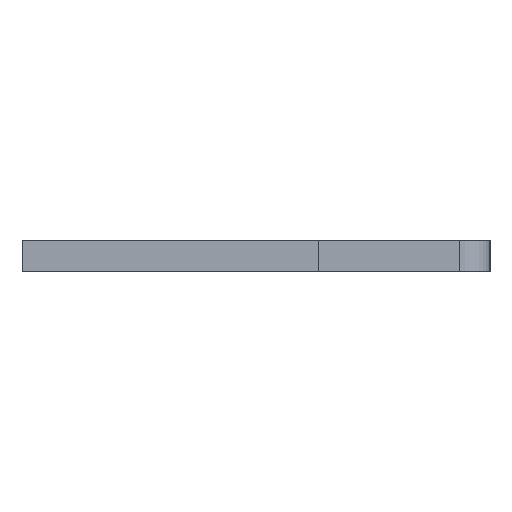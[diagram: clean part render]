
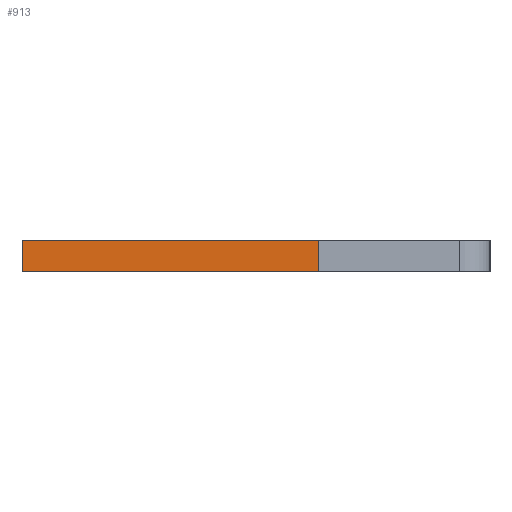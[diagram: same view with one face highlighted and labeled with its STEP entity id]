
A CAD part, left-side view. The second image highlights one B-rep face of the part: STEP entity #913.
In plain terms, the highlighted face is planar.
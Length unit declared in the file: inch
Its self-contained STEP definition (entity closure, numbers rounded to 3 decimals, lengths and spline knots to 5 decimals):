
#7 = CARTESIAN_POINT ( 'NONE',  ( 0.01, 0.15, -0.04 ) ) ;
#19 = DIRECTION ( 'NONE',  ( 1., 0., 0. ) ) ;
#22 = FACE_OUTER_BOUND ( 'NONE', #1101, .T. ) ;
#26 = VECTOR ( 'NONE', #312, 39.37008 ) ;
#32 = CARTESIAN_POINT ( 'NONE',  ( 0.01, 0.15, -0.04 ) ) ;
#194 = CARTESIAN_POINT ( 'NONE',  ( 0.01, 0.15, -0.04 ) ) ;
#196 = VECTOR ( 'NONE', #748, 39.37008 ) ;
#201 = CARTESIAN_POINT ( 'NONE',  ( 0.01, 0.15, -0.04 ) ) ;
#223 = PLANE ( 'NONE',  #752 ) ;
#224 = VECTOR ( 'NONE', #465, 39.37008 ) ;
#312 = DIRECTION ( 'NONE',  ( -1., 0., 0. ) ) ;
#334 = LINE ( 'NONE', #201, #196 ) ;
#358 = ORIENTED_EDGE ( 'NONE', *, *, #458, .T. ) ;
#382 = DIRECTION ( 'NONE',  ( 0., 1., 0. ) ) ;
#408 = VERTEX_POINT ( 'NONE', #848 ) ;
#410 = VECTOR ( 'NONE', #382, 39.37008 ) ;
#425 = VERTEX_POINT ( 'NONE', #737 ) ;
#458 = EDGE_CURVE ( 'NONE', #844, #408, #854, .T. ) ;
#465 = DIRECTION ( 'NONE',  ( 0., 1., 0. ) ) ;
#588 = DIRECTION ( 'NONE',  ( 0., 0., 1. ) ) ;
#610 = EDGE_CURVE ( 'NONE', #778, #425, #334, .T. ) ;
#670 = ORIENTED_EDGE ( 'NONE', *, *, #1131, .F. ) ;
#737 = CARTESIAN_POINT ( 'NONE',  ( -0.01, 0.15, -0.04 ) ) ;
#748 = DIRECTION ( 'NONE',  ( -1., 0., 0. ) ) ;
#750 = CARTESIAN_POINT ( 'NONE',  ( -0.01, 0.15, -0.04 ) ) ;
#752 = AXIS2_PLACEMENT_3D ( 'NONE', #32, #588, #19 ) ;
#778 = VERTEX_POINT ( 'NONE', #194 ) ;
#818 = ORIENTED_EDGE ( 'NONE', *, *, #610, .F. ) ;
#844 = VERTEX_POINT ( 'NONE', #877 ) ;
#848 = CARTESIAN_POINT ( 'NONE',  ( -0.01, -0.04, -0.04 ) ) ;
#854 = LINE ( 'NONE', #947, #26 ) ;
#871 = LINE ( 'NONE', #7, #224 ) ;
#877 = CARTESIAN_POINT ( 'NONE',  ( 0.01, -0.04, -0.04 ) ) ;
#913 = ADVANCED_FACE ( 'NONE', ( #22 ), #223, .F. ) ;
#947 = CARTESIAN_POINT ( 'NONE',  ( 0.01, -0.04, -0.04 ) ) ;
#1101 = EDGE_LOOP ( 'NONE', ( #1179, #818, #670, #358 ) ) ;
#1109 = LINE ( 'NONE', #750, #410 ) ;
#1131 = EDGE_CURVE ( 'NONE', #844, #778, #871, .T. ) ;
#1179 = ORIENTED_EDGE ( 'NONE', *, *, #1232, .T. ) ;
#1232 = EDGE_CURVE ( 'NONE', #408, #425, #1109, .T. ) ;
